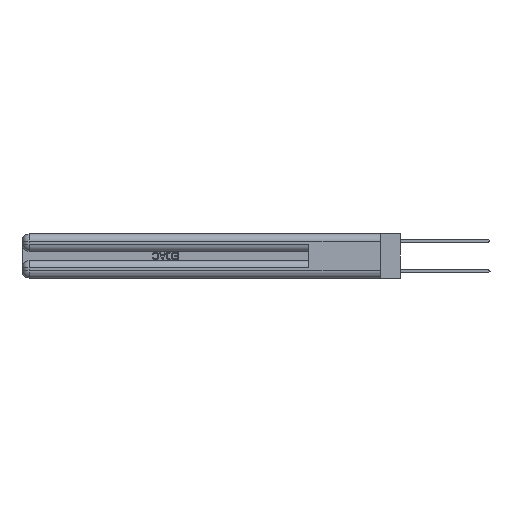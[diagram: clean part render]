
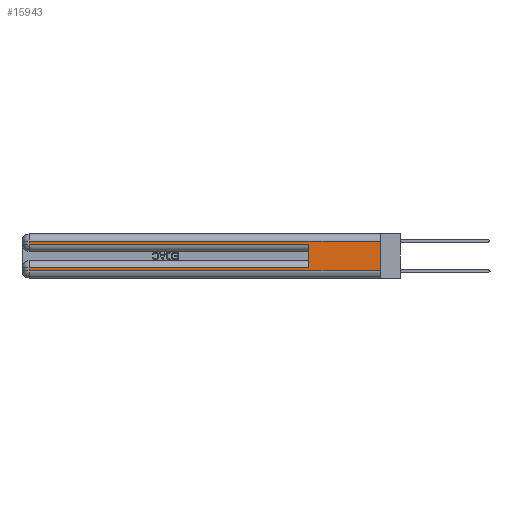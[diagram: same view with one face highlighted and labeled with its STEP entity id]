
A CAD part, left-side view. The second image highlights one B-rep face of the part: STEP entity #15943.
In plain terms, the highlighted planar face has unit normal (-1, 0, 0).
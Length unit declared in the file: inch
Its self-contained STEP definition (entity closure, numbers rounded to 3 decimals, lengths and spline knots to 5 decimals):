
#658 = LINE ( 'NONE', #29167, #6213 ) ;
#821 = AXIS2_PLACEMENT_3D ( 'NONE', #7782, #24462, #10181 ) ;
#1251 = VECTOR ( 'NONE', #12718, 39.37008 ) ;
#1872 = VERTEX_POINT ( 'NONE', #15283 ) ;
#1915 = EDGE_CURVE ( 'NONE', #28715, #2241, #4669, .T. ) ;
#2241 = VERTEX_POINT ( 'NONE', #23748 ) ;
#2765 = FACE_OUTER_BOUND ( 'NONE', #22928, .T. ) ;
#2788 = CARTESIAN_POINT ( 'NONE',  ( 0., 0., 0.06 ) ) ;
#3116 = DIRECTION ( 'NONE',  ( 0., 0., 1. ) ) ;
#3450 = CARTESIAN_POINT ( 'NONE',  ( 0., 0., 0.285 ) ) ;
#4247 = CARTESIAN_POINT ( 'NONE',  ( 0., 2.94, 0.285 ) ) ;
#4251 = EDGE_CURVE ( 'NONE', #9696, #14639, #24030, .T. ) ;
#4447 = DIRECTION ( 'NONE',  ( 0., 1., 0. ) ) ;
#4549 = VECTOR ( 'NONE', #8163, 39.37008 ) ;
#4669 = LINE ( 'NONE', #15389, #16583 ) ;
#5806 = ORIENTED_EDGE ( 'NONE', *, *, #28751, .T. ) ;
#6213 = VECTOR ( 'NONE', #3116, 39.37008 ) ;
#6443 = EDGE_CURVE ( 'NONE', #28685, #30193, #17205, .T. ) ;
#7782 = CARTESIAN_POINT ( 'NONE',  ( 0., 0., 0.37 ) ) ;
#7989 = ORIENTED_EDGE ( 'NONE', *, *, #6443, .T. ) ;
#8163 = DIRECTION ( 'NONE',  ( 0., 0., -1. ) ) ;
#9696 = VERTEX_POINT ( 'NONE', #22487 ) ;
#10181 = DIRECTION ( 'NONE',  ( 0., 0., -1. ) ) ;
#10219 = EDGE_CURVE ( 'NONE', #1872, #28685, #29810, .T. ) ;
#12718 = DIRECTION ( 'NONE',  ( 0., -1., 0. ) ) ;
#12990 = DIRECTION ( 'NONE',  ( 0., 1., 0. ) ) ;
#13229 = CARTESIAN_POINT ( 'NONE',  ( 0., 0., 0.37 ) ) ;
#13438 = VECTOR ( 'NONE', #4447, 39.37008 ) ;
#13771 = VECTOR ( 'NONE', #12990, 39.37008 ) ;
#13815 = CARTESIAN_POINT ( 'NONE',  ( 0., 2.94, 0.085 ) ) ;
#14639 = VERTEX_POINT ( 'NONE', #2788 ) ;
#14918 = PLANE ( 'NONE',  #821 ) ;
#15283 = CARTESIAN_POINT ( 'NONE',  ( 0., 2.94, 0.31 ) ) ;
#15389 = CARTESIAN_POINT ( 'NONE',  ( 0., 2.94, 0.37 ) ) ;
#15943 = ADVANCED_FACE ( 'NONE', ( #2765 ), #14918, .F. ) ;
#16134 = CARTESIAN_POINT ( 'NONE',  ( 0., 0.6, 0.285 ) ) ;
#16348 = ORIENTED_EDGE ( 'NONE', *, *, #20307, .T. ) ;
#16583 = VECTOR ( 'NONE', #22552, 39.37008 ) ;
#17205 = LINE ( 'NONE', #3450, #29055 ) ;
#17796 = ORIENTED_EDGE ( 'NONE', *, *, #24002, .F. ) ;
#17884 = EDGE_CURVE ( 'NONE', #2241, #14639, #26532, .T. ) ;
#18720 = CARTESIAN_POINT ( 'NONE',  ( 0., 0., 0.085 ) ) ;
#20104 = DIRECTION ( 'NONE',  ( 0., -1., 0. ) ) ;
#20118 = LINE ( 'NONE', #27246, #13771 ) ;
#20299 = VERTEX_POINT ( 'NONE', #22371 ) ;
#20307 = EDGE_CURVE ( 'NONE', #9696, #1872, #20118, .T. ) ;
#20525 = LINE ( 'NONE', #18720, #13438 ) ;
#20811 = ORIENTED_EDGE ( 'NONE', *, *, #10219, .T. ) ;
#21351 = ORIENTED_EDGE ( 'NONE', *, *, #1915, .T. ) ;
#22371 = CARTESIAN_POINT ( 'NONE',  ( 0., 0.6, 0.085 ) ) ;
#22487 = CARTESIAN_POINT ( 'NONE',  ( 0., 0., 0.31 ) ) ;
#22552 = DIRECTION ( 'NONE',  ( 0., 0., -1. ) ) ;
#22928 = EDGE_LOOP ( 'NONE', ( #26566, #16348, #20811, #7989, #17796, #5806, #21351, #28007 ) ) ;
#23748 = CARTESIAN_POINT ( 'NONE',  ( 0., 2.94, 0.06 ) ) ;
#24002 = EDGE_CURVE ( 'NONE', #20299, #30193, #658, .T. ) ;
#24030 = LINE ( 'NONE', #13229, #29564 ) ;
#24462 = DIRECTION ( 'NONE',  ( 1., 0., 0. ) ) ;
#24847 = CARTESIAN_POINT ( 'NONE',  ( 0., 2.94, 0.37 ) ) ;
#26532 = LINE ( 'NONE', #29298, #1251 ) ;
#26566 = ORIENTED_EDGE ( 'NONE', *, *, #4251, .F. ) ;
#27246 = CARTESIAN_POINT ( 'NONE',  ( 0., 0., 0.31 ) ) ;
#28007 = ORIENTED_EDGE ( 'NONE', *, *, #17884, .T. ) ;
#28685 = VERTEX_POINT ( 'NONE', #4247 ) ;
#28715 = VERTEX_POINT ( 'NONE', #13815 ) ;
#28751 = EDGE_CURVE ( 'NONE', #20299, #28715, #20525, .T. ) ;
#29055 = VECTOR ( 'NONE', #20104, 39.37008 ) ;
#29167 = CARTESIAN_POINT ( 'NONE',  ( 0., 0.6, 0.145 ) ) ;
#29298 = CARTESIAN_POINT ( 'NONE',  ( 0., 0., 0.06 ) ) ;
#29564 = VECTOR ( 'NONE', #29702, 39.37008 ) ;
#29702 = DIRECTION ( 'NONE',  ( 0., 0., -1. ) ) ;
#29810 = LINE ( 'NONE', #24847, #4549 ) ;
#30193 = VERTEX_POINT ( 'NONE', #16134 ) ;
